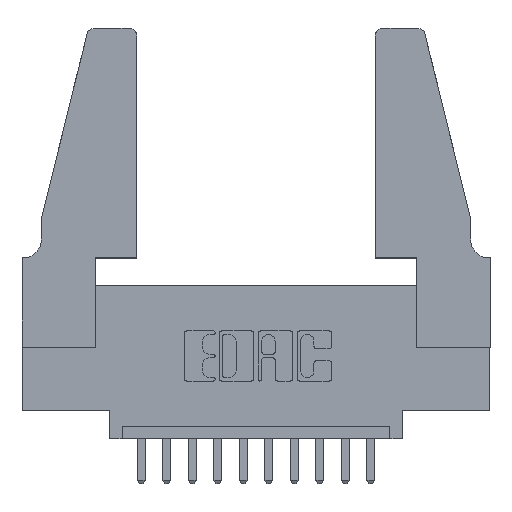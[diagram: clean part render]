
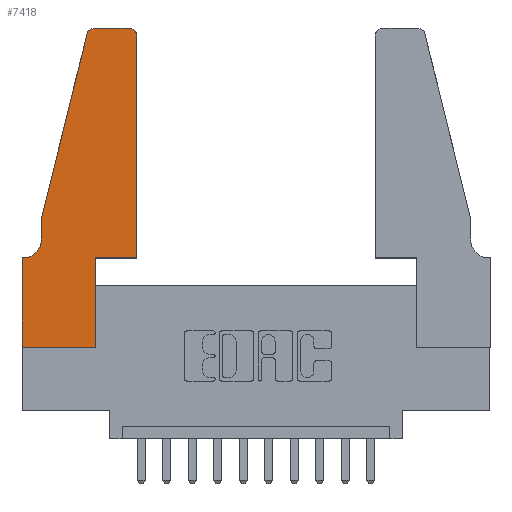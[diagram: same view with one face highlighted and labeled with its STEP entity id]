
A CAD part, top view. The second image highlights one B-rep face of the part: STEP entity #7418.
In plain terms, the highlighted planar face has unit normal (0, 0, 1).
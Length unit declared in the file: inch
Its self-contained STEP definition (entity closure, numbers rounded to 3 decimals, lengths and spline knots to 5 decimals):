
#461 = ORIENTED_EDGE ( 'NONE', *, *, #1959, .T. ) ;
#539 = CARTESIAN_POINT ( 'NONE',  ( 0., 0., 0.37 ) ) ;
#724 = EDGE_CURVE ( 'NONE', #7618, #1943, #3619, .T. ) ;
#928 = EDGE_CURVE ( 'NONE', #13942, #6170, #11533, .T. ) ;
#995 = VERTEX_POINT ( 'NONE', #11934 ) ;
#996 = CARTESIAN_POINT ( 'NONE',  ( 0.4505, 0.35, 0.37 ) ) ;
#1122 = CARTESIAN_POINT ( 'NONE',  ( 0.4205, 1.25, 0.37 ) ) ;
#1357 = ORIENTED_EDGE ( 'NONE', *, *, #7469, .T. ) ;
#1467 = VERTEX_POINT ( 'NONE', #12262 ) ;
#1553 = CIRCLE ( 'NONE', #4368, 0.03 ) ;
#1898 = DIRECTION ( 'NONE',  ( -0.239, -0.971, 0. ) ) ;
#1943 = VERTEX_POINT ( 'NONE', #1122 ) ;
#1959 = EDGE_CURVE ( 'NONE', #2355, #995, #1553, .T. ) ;
#2108 = CARTESIAN_POINT ( 'NONE',  ( 0.284, 1.25, 0.37 ) ) ;
#2355 = VERTEX_POINT ( 'NONE', #2108 ) ;
#2496 = DIRECTION ( 'NONE',  ( -1., 0., 0. ) ) ;
#2534 = LINE ( 'NONE', #13906, #10077 ) ;
#2555 = LINE ( 'NONE', #3845, #13891 ) ;
#2560 = VERTEX_POINT ( 'NONE', #7990 ) ;
#2638 = CARTESIAN_POINT ( 'NONE',  ( 0., 0., 0.37 ) ) ;
#2713 = AXIS2_PLACEMENT_3D ( 'NONE', #7243, #7442, #12756 ) ;
#2731 = EDGE_CURVE ( 'NONE', #10344, #2560, #2555, .T. ) ;
#2745 = DIRECTION ( 'NONE',  ( 0., -1., 0. ) ) ;
#2985 = VERTEX_POINT ( 'NONE', #6732 ) ;
#3151 = EDGE_CURVE ( 'NONE', #3601, #7376, #12656, .T. ) ;
#3198 = DIRECTION ( 'NONE',  ( 1., 0., 0. ) ) ;
#3215 = EDGE_CURVE ( 'NONE', #1943, #2355, #11296, .T. ) ;
#3516 = EDGE_LOOP ( 'NONE', ( #4449, #461, #12688, #9836, #11438, #12924, #11491, #11960, #6136, #12143, #1357, #10982 ) ) ;
#3601 = VERTEX_POINT ( 'NONE', #5362 ) ;
#3619 = CIRCLE ( 'NONE', #2713, 0.03 ) ;
#3640 = VECTOR ( 'NONE', #2496, 39.37008 ) ;
#3845 = CARTESIAN_POINT ( 'NONE',  ( 0.0755, 0.5, 0.37 ) ) ;
#3922 = AXIS2_PLACEMENT_3D ( 'NONE', #14033, #4273, #10857 ) ;
#4273 = DIRECTION ( 'NONE',  ( 0., 0., -1. ) ) ;
#4368 = AXIS2_PLACEMENT_3D ( 'NONE', #5560, #11059, #8774 ) ;
#4406 = EDGE_CURVE ( 'NONE', #2560, #1467, #6477, .T. ) ;
#4449 = ORIENTED_EDGE ( 'NONE', *, *, #3215, .T. ) ;
#4506 = LINE ( 'NONE', #9060, #3640 ) ;
#4752 = CARTESIAN_POINT ( 'NONE',  ( 0., 0.35, 0.37 ) ) ;
#4756 = CARTESIAN_POINT ( 'NONE',  ( 0.2865, 0.35, 0.37 ) ) ;
#5125 = DIRECTION ( 'NONE',  ( 1., 0., 0. ) ) ;
#5162 = AXIS2_PLACEMENT_3D ( 'NONE', #4752, #13666, #9329 ) ;
#5362 = CARTESIAN_POINT ( 'NONE',  ( 0., 0.35, 0.37 ) ) ;
#5560 = CARTESIAN_POINT ( 'NONE',  ( 0.284, 1.22, 0.37 ) ) ;
#5713 = LINE ( 'NONE', #13630, #8615 ) ;
#5920 = CARTESIAN_POINT ( 'NONE',  ( 0.4505, 1.22, 0.37 ) ) ;
#5971 = DIRECTION ( 'NONE',  ( -1., 0., 0. ) ) ;
#6015 = EDGE_CURVE ( 'NONE', #6170, #2985, #13436, .T. ) ;
#6084 = DIRECTION ( 'NONE',  ( 0., -1., 0. ) ) ;
#6136 = ORIENTED_EDGE ( 'NONE', *, *, #928, .T. ) ;
#6138 = EDGE_CURVE ( 'NONE', #1467, #3601, #4506, .T. ) ;
#6170 = VERTEX_POINT ( 'NONE', #4756 ) ;
#6477 = CIRCLE ( 'NONE', #3922, 0.07 ) ;
#6732 = CARTESIAN_POINT ( 'NONE',  ( 0.4505, 0.35, 0.37 ) ) ;
#7243 = CARTESIAN_POINT ( 'NONE',  ( 0.4205, 1.22, 0.37 ) ) ;
#7263 = VECTOR ( 'NONE', #3198, 39.37008 ) ;
#7376 = VERTEX_POINT ( 'NONE', #539 ) ;
#7403 = CARTESIAN_POINT ( 'NONE',  ( 0.2865, 0.35, 0.37 ) ) ;
#7418 = ADVANCED_FACE ( 'NONE', ( #12024 ), #9054, .T. ) ;
#7442 = DIRECTION ( 'NONE',  ( 0., 0., 1. ) ) ;
#7469 = EDGE_CURVE ( 'NONE', #2985, #7618, #2534, .T. ) ;
#7526 = CARTESIAN_POINT ( 'NONE',  ( 0.0755, 0.5, 0.37 ) ) ;
#7618 = VERTEX_POINT ( 'NONE', #5920 ) ;
#7990 = CARTESIAN_POINT ( 'NONE',  ( 0.0755, 0.42, 0.37 ) ) ;
#8095 = EDGE_CURVE ( 'NONE', #7376, #13942, #13325, .T. ) ;
#8194 = VECTOR ( 'NONE', #2745, 39.37008 ) ;
#8330 = DIRECTION ( 'NONE',  ( 0., 1., 0. ) ) ;
#8615 = VECTOR ( 'NONE', #1898, 39.37008 ) ;
#8774 = DIRECTION ( 'NONE',  ( 1., 0., 0. ) ) ;
#9054 = PLANE ( 'NONE',  #5162 ) ;
#9060 = CARTESIAN_POINT ( 'NONE',  ( 0.0755, 0.35, 0.37 ) ) ;
#9153 = CARTESIAN_POINT ( 'NONE',  ( 0.2605, 1.25, 0.37 ) ) ;
#9329 = DIRECTION ( 'NONE',  ( 1., 0., 0. ) ) ;
#9451 = CARTESIAN_POINT ( 'NONE',  ( 0., 0., 0.37 ) ) ;
#9484 = DIRECTION ( 'NONE',  ( 0., 1., 0. ) ) ;
#9777 = VECTOR ( 'NONE', #9484, 39.37008 ) ;
#9836 = ORIENTED_EDGE ( 'NONE', *, *, #2731, .T. ) ;
#10077 = VECTOR ( 'NONE', #8330, 39.37008 ) ;
#10344 = VERTEX_POINT ( 'NONE', #7526 ) ;
#10857 = DIRECTION ( 'NONE',  ( -1., 0., 0. ) ) ;
#10982 = ORIENTED_EDGE ( 'NONE', *, *, #724, .T. ) ;
#11059 = DIRECTION ( 'NONE',  ( 0., 0., 1. ) ) ;
#11296 = LINE ( 'NONE', #9153, #12171 ) ;
#11423 = EDGE_CURVE ( 'NONE', #995, #10344, #5713, .T. ) ;
#11438 = ORIENTED_EDGE ( 'NONE', *, *, #4406, .T. ) ;
#11491 = ORIENTED_EDGE ( 'NONE', *, *, #3151, .T. ) ;
#11533 = LINE ( 'NONE', #7403, #9777 ) ;
#11934 = CARTESIAN_POINT ( 'NONE',  ( 0.25487, 1.22718, 0.37 ) ) ;
#11960 = ORIENTED_EDGE ( 'NONE', *, *, #8095, .T. ) ;
#12024 = FACE_OUTER_BOUND ( 'NONE', #3516, .T. ) ;
#12143 = ORIENTED_EDGE ( 'NONE', *, *, #6015, .T. ) ;
#12171 = VECTOR ( 'NONE', #5971, 39.37008 ) ;
#12262 = CARTESIAN_POINT ( 'NONE',  ( 0.0055, 0.35, 0.37 ) ) ;
#12656 = LINE ( 'NONE', #2638, #8194 ) ;
#12688 = ORIENTED_EDGE ( 'NONE', *, *, #11423, .T. ) ;
#12756 = DIRECTION ( 'NONE',  ( 1., 0., 0. ) ) ;
#12784 = CARTESIAN_POINT ( 'NONE',  ( 0.2865, 0., 0.37 ) ) ;
#12924 = ORIENTED_EDGE ( 'NONE', *, *, #6138, .T. ) ;
#13325 = LINE ( 'NONE', #9451, #13502 ) ;
#13436 = LINE ( 'NONE', #996, #7263 ) ;
#13502 = VECTOR ( 'NONE', #5125, 39.37008 ) ;
#13630 = CARTESIAN_POINT ( 'NONE',  ( 0.0755, 0.5, 0.37 ) ) ;
#13666 = DIRECTION ( 'NONE',  ( 0., 0., 1. ) ) ;
#13891 = VECTOR ( 'NONE', #6084, 39.37008 ) ;
#13906 = CARTESIAN_POINT ( 'NONE',  ( 0.4505, 0.35, 0.37 ) ) ;
#13942 = VERTEX_POINT ( 'NONE', #12784 ) ;
#14033 = CARTESIAN_POINT ( 'NONE',  ( 0.0055, 0.42, 0.37 ) ) ;
